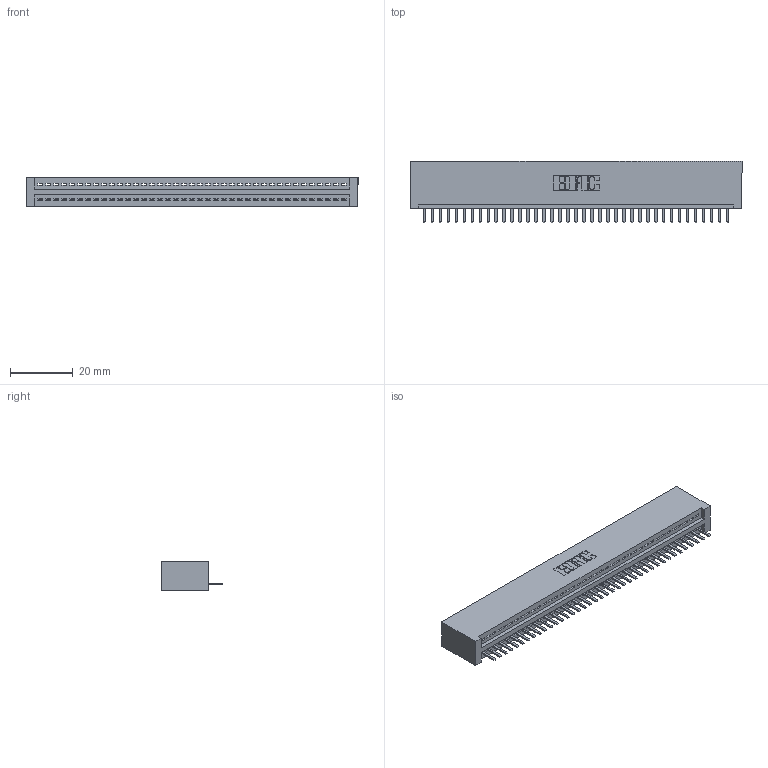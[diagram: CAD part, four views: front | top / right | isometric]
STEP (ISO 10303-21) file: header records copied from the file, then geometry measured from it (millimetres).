
FILE_DESCRIPTION (( 'STEP AP203' ), '1' );
FILE_NAME ('395-039-520-101.STEP', '2018-11-14T07:52:41', ( '' ), ( '' ), 'SwSTEP 2.0', 'SolidWorks 2016', '' );
FILE_SCHEMA (( 'CONFIG_CONTROL_DESIGN' ));
Length unit declared in the file: inch
Products named in the file (3): 395-039-520-101; 345 Part_No Mounting Lugs; 345-292-001_345-293-120
Assembly tree (40 placements, depth 2):
  395-039-520-101
    345 Part_No Mounting Lugs
    345-292-001_345-293-120  x39
Bounding box: 105.66 x 19.68 x 9.4 mm (x, y, z)
Volume: 10483.7 mm3; surface area: 13714.2 mm2
Topology: 40 solids, 40 shells, 2536 faces, 7493 edges, 4890 vertices
Faces by surface type: plane 1714, cylinder 822
Entity records: 29593 total; most frequent: CARTESIAN_POINT 5145, ORIENTED_EDGE 5106, DIRECTION 4479, EDGE_CURVE 2553, LINE 2269, VECTOR 2269, VERTEX_POINT 1698, AXIS2_PLACEMENT_3D 1105
